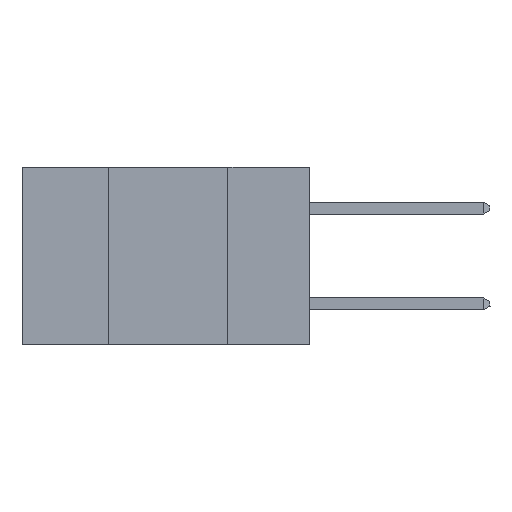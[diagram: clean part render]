
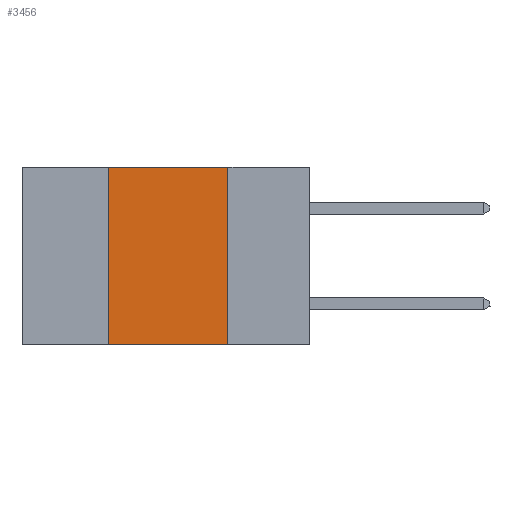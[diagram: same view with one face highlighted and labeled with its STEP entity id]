
A CAD part, left-side view. The second image highlights one B-rep face of the part: STEP entity #3456.
In plain terms, the highlighted planar face has unit normal (-1, 0, 0).
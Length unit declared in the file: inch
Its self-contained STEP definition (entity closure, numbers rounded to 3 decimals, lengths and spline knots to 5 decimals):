
#406 = CARTESIAN_POINT ( 'NONE',  ( 0., 0.17, -0.37 ) ) ;
#1057 = CARTESIAN_POINT ( 'NONE',  ( 0., 0.42, -0.37 ) ) ;
#1391 = CARTESIAN_POINT ( 'NONE',  ( 0., 0.42, 0. ) ) ;
#1944 = LINE ( 'NONE', #11086, #11240 ) ;
#2661 = CARTESIAN_POINT ( 'NONE',  ( 0., 0.17, 0. ) ) ;
#3205 = EDGE_CURVE ( 'NONE', #11334, #13878, #17343, .T. ) ;
#3456 = ADVANCED_FACE ( 'NONE', ( #5529 ), #19222, .F. ) ;
#4407 = ORIENTED_EDGE ( 'NONE', *, *, #17153, .F. ) ;
#4675 = LINE ( 'NONE', #20959, #10253 ) ;
#5529 = FACE_OUTER_BOUND ( 'NONE', #14441, .T. ) ;
#5735 = ORIENTED_EDGE ( 'NONE', *, *, #22600, .F. ) ;
#7040 = DIRECTION ( 'NONE',  ( 0., -1., 0. ) ) ;
#7123 = EDGE_CURVE ( 'NONE', #11334, #18728, #4675, .T. ) ;
#7363 = CARTESIAN_POINT ( 'NONE',  ( 0., 0.6, 0. ) ) ;
#7697 = AXIS2_PLACEMENT_3D ( 'NONE', #7363, #13201, #21398 ) ;
#8924 = DIRECTION ( 'NONE',  ( 0., 0., 1. ) ) ;
#10253 = VECTOR ( 'NONE', #8924, 39.37008 ) ;
#10615 = CARTESIAN_POINT ( 'NONE',  ( 0., 0.6, -0.37 ) ) ;
#11086 = CARTESIAN_POINT ( 'NONE',  ( 0., 0.17, 0. ) ) ;
#11089 = CARTESIAN_POINT ( 'NONE',  ( 0., 0.6, 0. ) ) ;
#11240 = VECTOR ( 'NONE', #23266, 39.37008 ) ;
#11334 = VERTEX_POINT ( 'NONE', #1057 ) ;
#12478 = ORIENTED_EDGE ( 'NONE', *, *, #7123, .F. ) ;
#13201 = DIRECTION ( 'NONE',  ( 1., 0., 0. ) ) ;
#13878 = VERTEX_POINT ( 'NONE', #406 ) ;
#14441 = EDGE_LOOP ( 'NONE', ( #4407, #5735, #12478, #21733 ) ) ;
#16544 = DIRECTION ( 'NONE',  ( 0., -1., 0. ) ) ;
#17153 = EDGE_CURVE ( 'NONE', #24255, #13878, #1944, .T. ) ;
#17343 = LINE ( 'NONE', #10615, #25554 ) ;
#17818 = VECTOR ( 'NONE', #7040, 39.37008 ) ;
#18728 = VERTEX_POINT ( 'NONE', #1391 ) ;
#19222 = PLANE ( 'NONE',  #7697 ) ;
#20954 = LINE ( 'NONE', #11089, #17818 ) ;
#20959 = CARTESIAN_POINT ( 'NONE',  ( 0., 0.42, 0. ) ) ;
#21398 = DIRECTION ( 'NONE',  ( 0., 0., -1. ) ) ;
#21733 = ORIENTED_EDGE ( 'NONE', *, *, #3205, .T. ) ;
#22600 = EDGE_CURVE ( 'NONE', #18728, #24255, #20954, .T. ) ;
#23266 = DIRECTION ( 'NONE',  ( 0., 0., -1. ) ) ;
#24255 = VERTEX_POINT ( 'NONE', #2661 ) ;
#25554 = VECTOR ( 'NONE', #16544, 39.37008 ) ;
